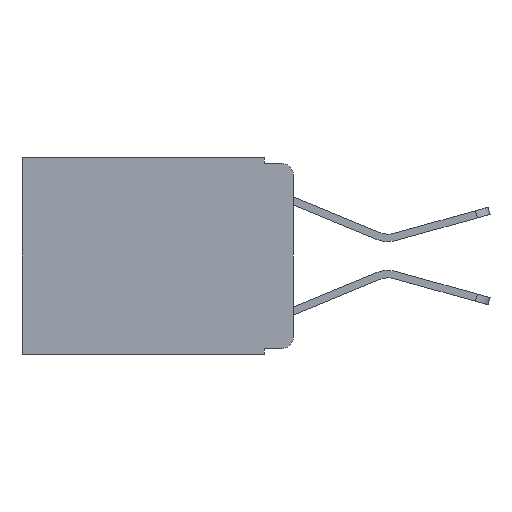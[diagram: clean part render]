
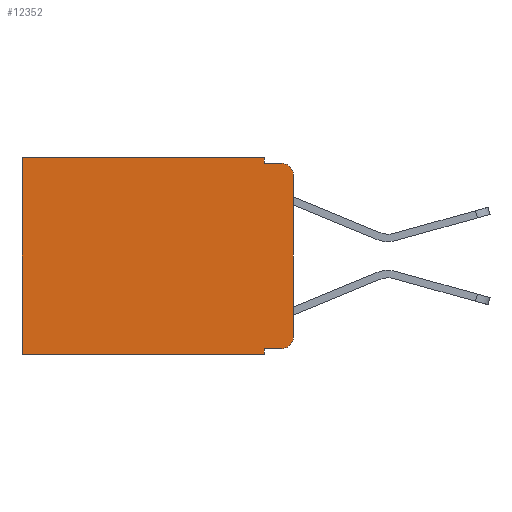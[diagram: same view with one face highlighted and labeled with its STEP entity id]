
A CAD part, left-side view. The second image highlights one B-rep face of the part: STEP entity #12352.
In plain terms, the highlighted planar face has unit normal (-1, 0, 0).
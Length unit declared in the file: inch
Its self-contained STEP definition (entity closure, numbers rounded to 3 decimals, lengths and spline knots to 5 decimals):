
#562 = EDGE_LOOP ( 'NONE', ( #16280, #8953, #9929, #7065, #16118, #1330, #11552, #1422, #10734, #5743 ) ) ;
#615 = CARTESIAN_POINT ( 'NONE',  ( 0.298, 0.473, 0. ) ) ;
#1025 = CIRCLE ( 'NONE', #7486, 0.02 ) ;
#1139 = VERTEX_POINT ( 'NONE', #8447 ) ;
#1153 = DIRECTION ( 'NONE',  ( 0., 0., -1. ) ) ;
#1276 = CARTESIAN_POINT ( 'NONE',  ( 0.298, 0.02, -0.03 ) ) ;
#1330 = ORIENTED_EDGE ( 'NONE', *, *, #2484, .T. ) ;
#1422 = ORIENTED_EDGE ( 'NONE', *, *, #16207, .F. ) ;
#1434 = VECTOR ( 'NONE', #15311, 39.37008 ) ;
#1595 = EDGE_CURVE ( 'NONE', #6451, #1139, #15580, .T. ) ;
#1659 = VERTEX_POINT ( 'NONE', #13351 ) ;
#1789 = LINE ( 'NONE', #14558, #11602 ) ;
#1848 = EDGE_CURVE ( 'NONE', #5929, #2712, #15385, .T. ) ;
#1963 = LINE ( 'NONE', #15975, #11773 ) ;
#2484 = EDGE_CURVE ( 'NONE', #1659, #6324, #11441, .T. ) ;
#2579 = DIRECTION ( 'NONE',  ( 0., 0., -1. ) ) ;
#2712 = VERTEX_POINT ( 'NONE', #11635 ) ;
#2977 = VECTOR ( 'NONE', #12045, 39.37008 ) ;
#3010 = EDGE_CURVE ( 'NONE', #3684, #1139, #6401, .T. ) ;
#3114 = DIRECTION ( 'NONE',  ( 0., -1., 0. ) ) ;
#3205 = DIRECTION ( 'NONE',  ( 0., 1., 0. ) ) ;
#3260 = DIRECTION ( 'NONE',  ( -1., 0., 0. ) ) ;
#3684 = VERTEX_POINT ( 'NONE', #16329 ) ;
#3858 = VECTOR ( 'NONE', #3205, 39.37008 ) ;
#4498 = EDGE_CURVE ( 'NONE', #2712, #8911, #4913, .T. ) ;
#4586 = VERTEX_POINT ( 'NONE', #8525 ) ;
#4913 = LINE ( 'NONE', #8588, #11365 ) ;
#5230 = CARTESIAN_POINT ( 'NONE',  ( 0.298, 0., 0. ) ) ;
#5743 = ORIENTED_EDGE ( 'NONE', *, *, #1595, .T. ) ;
#5850 = VERTEX_POINT ( 'NONE', #6983 ) ;
#5929 = VERTEX_POINT ( 'NONE', #13080 ) ;
#6266 = AXIS2_PLACEMENT_3D ( 'NONE', #14703, #3260, #1153 ) ;
#6324 = VERTEX_POINT ( 'NONE', #13409 ) ;
#6401 = LINE ( 'NONE', #12383, #2977 ) ;
#6451 = VERTEX_POINT ( 'NONE', #15297 ) ;
#6587 = DIRECTION ( 'NONE',  ( 1., 0., 0. ) ) ;
#6983 = CARTESIAN_POINT ( 'NONE',  ( 0.298, 0.051, -0.333 ) ) ;
#7065 = ORIENTED_EDGE ( 'NONE', *, *, #1848, .F. ) ;
#7363 = DIRECTION ( 'NONE',  ( 0., -1., 0. ) ) ;
#7486 = AXIS2_PLACEMENT_3D ( 'NONE', #1276, #10277, #2579 ) ;
#8031 = VECTOR ( 'NONE', #15606, 39.37008 ) ;
#8247 = CARTESIAN_POINT ( 'NONE',  ( 0.298, 0.051, -0.333 ) ) ;
#8447 = CARTESIAN_POINT ( 'NONE',  ( 0.298, 0., -0.313 ) ) ;
#8525 = CARTESIAN_POINT ( 'NONE',  ( 0.298, 0.051, -0.343 ) ) ;
#8588 = CARTESIAN_POINT ( 'NONE',  ( 0.298, 0.051, -0.01 ) ) ;
#8780 = VECTOR ( 'NONE', #3114, 39.37008 ) ;
#8911 = VERTEX_POINT ( 'NONE', #13676 ) ;
#8953 = ORIENTED_EDGE ( 'NONE', *, *, #12244, .T. ) ;
#9357 = EDGE_CURVE ( 'NONE', #5850, #6451, #12530, .T. ) ;
#9929 = ORIENTED_EDGE ( 'NONE', *, *, #4498, .F. ) ;
#10277 = DIRECTION ( 'NONE',  ( -1., 0., 0. ) ) ;
#10643 = EDGE_CURVE ( 'NONE', #5929, #1659, #13640, .T. ) ;
#10734 = ORIENTED_EDGE ( 'NONE', *, *, #9357, .T. ) ;
#10930 = CARTESIAN_POINT ( 'NONE',  ( 0.298, 0., 0. ) ) ;
#11365 = VECTOR ( 'NONE', #7363, 39.37008 ) ;
#11441 = LINE ( 'NONE', #615, #8031 ) ;
#11552 = ORIENTED_EDGE ( 'NONE', *, *, #15595, .F. ) ;
#11602 = VECTOR ( 'NONE', #15798, 39.37008 ) ;
#11635 = CARTESIAN_POINT ( 'NONE',  ( 0.298, 0.051, -0.01 ) ) ;
#11773 = VECTOR ( 'NONE', #12210, 39.37008 ) ;
#11833 = FACE_OUTER_BOUND ( 'NONE', #562, .T. ) ;
#12045 = DIRECTION ( 'NONE',  ( 0., 0., -1. ) ) ;
#12210 = DIRECTION ( 'NONE',  ( 0., 0., -1. ) ) ;
#12244 = EDGE_CURVE ( 'NONE', #3684, #8911, #1025, .T. ) ;
#12352 = ADVANCED_FACE ( 'NONE', ( #11833 ), #14224, .F. ) ;
#12383 = CARTESIAN_POINT ( 'NONE',  ( 0.298, 0., 0. ) ) ;
#12530 = LINE ( 'NONE', #8247, #8780 ) ;
#13080 = CARTESIAN_POINT ( 'NONE',  ( 0.298, 0.051, 0. ) ) ;
#13351 = CARTESIAN_POINT ( 'NONE',  ( 0.298, 0.473, 0. ) ) ;
#13409 = CARTESIAN_POINT ( 'NONE',  ( 0.298, 0.473, -0.343 ) ) ;
#13640 = LINE ( 'NONE', #10930, #3858 ) ;
#13676 = CARTESIAN_POINT ( 'NONE',  ( 0.298, 0.02, -0.01 ) ) ;
#14224 = PLANE ( 'NONE',  #15960 ) ;
#14541 = CARTESIAN_POINT ( 'NONE',  ( 0.298, 0.051, 0. ) ) ;
#14558 = CARTESIAN_POINT ( 'NONE',  ( 0.298, 0., -0.343 ) ) ;
#14703 = CARTESIAN_POINT ( 'NONE',  ( 0.298, 0.02, -0.313 ) ) ;
#15297 = CARTESIAN_POINT ( 'NONE',  ( 0.298, 0.02, -0.333 ) ) ;
#15311 = DIRECTION ( 'NONE',  ( 0., 0., -1. ) ) ;
#15385 = LINE ( 'NONE', #14541, #1434 ) ;
#15480 = DIRECTION ( 'NONE',  ( 0., 0., -1. ) ) ;
#15580 = CIRCLE ( 'NONE', #6266, 0.02 ) ;
#15595 = EDGE_CURVE ( 'NONE', #4586, #6324, #1789, .T. ) ;
#15606 = DIRECTION ( 'NONE',  ( 0., 0., -1. ) ) ;
#15798 = DIRECTION ( 'NONE',  ( 0., 1., 0. ) ) ;
#15960 = AXIS2_PLACEMENT_3D ( 'NONE', #5230, #6587, #15480 ) ;
#15975 = CARTESIAN_POINT ( 'NONE',  ( 0.298, 0.051, 0. ) ) ;
#16118 = ORIENTED_EDGE ( 'NONE', *, *, #10643, .T. ) ;
#16207 = EDGE_CURVE ( 'NONE', #5850, #4586, #1963, .T. ) ;
#16280 = ORIENTED_EDGE ( 'NONE', *, *, #3010, .F. ) ;
#16329 = CARTESIAN_POINT ( 'NONE',  ( 0.298, 0., -0.03 ) ) ;
